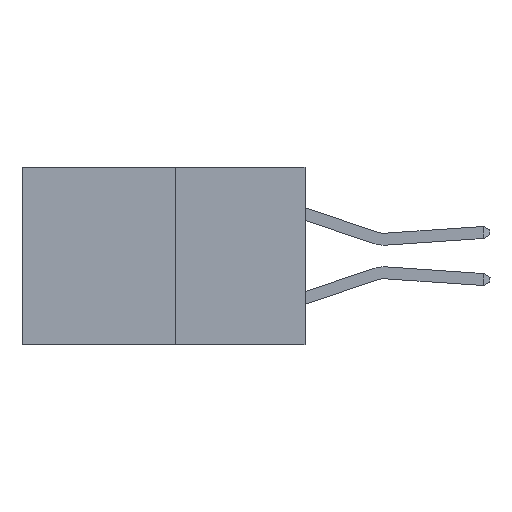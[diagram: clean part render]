
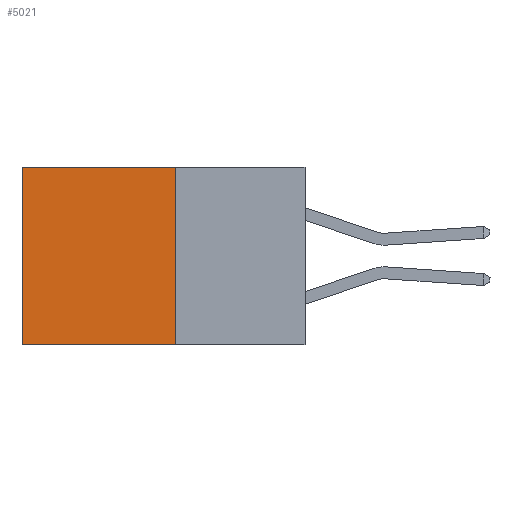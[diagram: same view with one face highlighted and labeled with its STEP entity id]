
A CAD part, left-side view. The second image highlights one B-rep face of the part: STEP entity #5021.
In plain terms, the highlighted planar face has unit normal (-1, 0, 0).
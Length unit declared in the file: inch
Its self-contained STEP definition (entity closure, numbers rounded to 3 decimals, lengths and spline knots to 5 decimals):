
#42 = AXIS2_PLACEMENT_3D ( 'NONE', #8664, #1684, #6607 ) ;
#231 = EDGE_LOOP ( 'NONE', ( #5278, #5305, #5342, #5602 ) ) ;
#1059 = VECTOR ( 'NONE', #2823, 39.37008 ) ;
#1190 = CARTESIAN_POINT ( 'NONE',  ( 0.277, 0.59, -0.37 ) ) ;
#1684 = DIRECTION ( 'NONE',  ( 1., 0., 0. ) ) ;
#2303 = CARTESIAN_POINT ( 'NONE',  ( 0.277, 0.27, -0.37 ) ) ;
#2823 = DIRECTION ( 'NONE',  ( 0., 1., 0. ) ) ;
#2896 = VERTEX_POINT ( 'NONE', #4317 ) ;
#3077 = VERTEX_POINT ( 'NONE', #5775 ) ;
#3467 = DIRECTION ( 'NONE',  ( 0., 0., -1. ) ) ;
#3628 = LINE ( 'NONE', #8308, #8863 ) ;
#3640 = VECTOR ( 'NONE', #7900, 39.37008 ) ;
#3920 = VERTEX_POINT ( 'NONE', #5807 ) ;
#4317 = CARTESIAN_POINT ( 'NONE',  ( 0.277, 0.27, 0. ) ) ;
#4493 = LINE ( 'NONE', #6975, #1059 ) ;
#4558 = VECTOR ( 'NONE', #3467, 39.37008 ) ;
#5021 = ADVANCED_FACE ( 'NONE', ( #6235 ), #7283, .F. ) ;
#5250 = VERTEX_POINT ( 'NONE', #5455 ) ;
#5278 = ORIENTED_EDGE ( 'NONE', *, *, #8670, .T. ) ;
#5305 = ORIENTED_EDGE ( 'NONE', *, *, #6601, .F. ) ;
#5342 = ORIENTED_EDGE ( 'NONE', *, *, #7674, .F. ) ;
#5455 = CARTESIAN_POINT ( 'NONE',  ( 0.277, 0.59, 0. ) ) ;
#5602 = ORIENTED_EDGE ( 'NONE', *, *, #8126, .T. ) ;
#5775 = CARTESIAN_POINT ( 'NONE',  ( 0.277, 0.27, -0.37 ) ) ;
#5807 = CARTESIAN_POINT ( 'NONE',  ( 0.277, 0.59, -0.37 ) ) ;
#6235 = FACE_OUTER_BOUND ( 'NONE', #231, .T. ) ;
#6591 = LINE ( 'NONE', #1190, #4558 ) ;
#6601 = EDGE_CURVE ( 'NONE', #3077, #3920, #4493, .T. ) ;
#6607 = DIRECTION ( 'NONE',  ( 0., 0., -1. ) ) ;
#6975 = CARTESIAN_POINT ( 'NONE',  ( 0.277, 0.27, -0.37 ) ) ;
#7283 = PLANE ( 'NONE',  #42 ) ;
#7674 = EDGE_CURVE ( 'NONE', #2896, #3077, #8666, .T. ) ;
#7900 = DIRECTION ( 'NONE',  ( 0., 0., -1. ) ) ;
#8126 = EDGE_CURVE ( 'NONE', #2896, #5250, #3628, .T. ) ;
#8308 = CARTESIAN_POINT ( 'NONE',  ( 0.277, 0.27, 0. ) ) ;
#8664 = CARTESIAN_POINT ( 'NONE',  ( 0.277, 0.27, -0.37 ) ) ;
#8666 = LINE ( 'NONE', #2303, #3640 ) ;
#8670 = EDGE_CURVE ( 'NONE', #5250, #3920, #6591, .T. ) ;
#8863 = VECTOR ( 'NONE', #8961, 39.37008 ) ;
#8961 = DIRECTION ( 'NONE',  ( 0., 1., 0. ) ) ;
